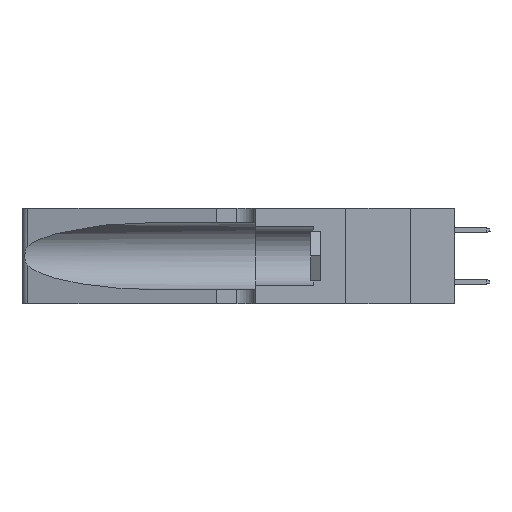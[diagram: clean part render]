
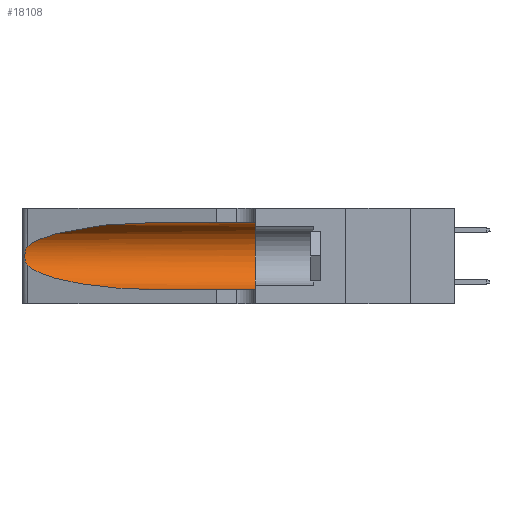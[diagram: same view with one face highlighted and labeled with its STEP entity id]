
A CAD part, left-side view. The second image highlights one B-rep face of the part: STEP entity #18108.
In plain terms, the highlighted cylindrical face has radius 3.308 mm (diameter 6.617 mm), a partial arc.
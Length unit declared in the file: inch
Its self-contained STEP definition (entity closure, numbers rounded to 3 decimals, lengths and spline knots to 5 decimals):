
#57 = CARTESIAN_POINT ( 'NONE',  ( 0.25487, 1.22718, 0.22369 ) ) ;
#286 = CARTESIAN_POINT ( 'NONE',  ( 0.26017, 1.23833, 0.17102 ) ) ;
#484 = CARTESIAN_POINT ( 'NONE',  ( 0.1305, 0.35, 0.31525 ) ) ;
#675 = ORIENTED_EDGE ( 'NONE', *, *, #28001, .F. ) ;
#751 = ORIENTED_EDGE ( 'NONE', *, *, #20551, .F. ) ;
#2755 = VERTEX_POINT ( 'NONE', #484 ) ;
#4154 = DIRECTION ( 'NONE',  ( 0., -1., 0. ) ) ;
#4269 = CARTESIAN_POINT ( 'NONE',  ( 0.25555, 1.22993, 0.14849 ) ) ;
#4335 = CARTESIAN_POINT ( 'NONE',  ( 0.1305, 0.72297, 0.05475 ) ) ;
#4946 = CARTESIAN_POINT ( 'NONE',  ( 0.25487, 1.22718, 0.14631 ) ) ;
#5287 = DIRECTION ( 'NONE',  ( 0., -1., 0. ) ) ;
#5870 = VERTEX_POINT ( 'NONE', #4335 ) ;
#6029 = CARTESIAN_POINT ( 'NONE',  ( 0.1305, 0.72297, 0.05475 ) ) ;
#6199 = CARTESIAN_POINT ( 'NONE',  ( 0.18966, 0.96281, 0.31525 ) ) ;
#7295 = CARTESIAN_POINT ( 'NONE',  ( 0.25854, 1.2359, 0.20912 ) ) ;
#7402 = ORIENTED_EDGE ( 'NONE', *, *, #29773, .T. ) ;
#7566 = DIRECTION ( 'NONE',  ( 0., -1., 0. ) ) ;
#8122 = VERTEX_POINT ( 'NONE', #38516 ) ;
#8570 = ORIENTED_EDGE ( 'NONE', *, *, #28626, .T. ) ;
#11115 = CYLINDRICAL_SURFACE ( 'NONE', #35770, 0.13025 ) ;
#11534 = EDGE_LOOP ( 'NONE', ( #14962, #7402, #8570, #28116, #751, #675 ) ) ;
#14216 = CARTESIAN_POINT ( 'NONE',  ( 0.25555, 1.22994, 0.2215 ) ) ;
#14439 = CARTESIAN_POINT ( 'NONE',  ( 0.25856, 1.23593, 0.16098 ) ) ;
#14962 = ORIENTED_EDGE ( 'NONE', *, *, #38275, .T. ) ;
#16842 = CARTESIAN_POINT ( 'NONE',  ( 0.2373, 1.15595, 0.28018 ) ) ;
#18108 = ADVANCED_FACE ( 'NONE', ( #24962 ), #11115, .F. ) ;
#18356 = CARTESIAN_POINT ( 'NONE',  ( 0.25639, 1.23186, 0.15144 ) ) ;
#20551 = EDGE_CURVE ( 'NONE', #2755, #45360, #32993, .T. ) ;
#21380 = CARTESIAN_POINT ( 'NONE',  ( 0.26018, 1.23835, 0.19895 ) ) ;
#22096 = LINE ( 'NONE', #28857, #41664 ) ;
#23373 = CARTESIAN_POINT ( 'NONE',  ( 0.25487, 1.22718, 0.14631 ) ) ;
#23606 = CARTESIAN_POINT ( 'NONE',  ( 0.18966, 0.96281, 0.05475 ) ) ;
#24962 = FACE_OUTER_BOUND ( 'NONE', #11534, .T. ) ;
#25114 = VECTOR ( 'NONE', #5287, 39.37008 ) ;
#25189 = CARTESIAN_POINT ( 'NONE',  ( 0.1305, 1.61858, 0.185 ) ) ;
#25211 = CARTESIAN_POINT ( 'NONE',  ( 0.1305, 0.35, 0.05475 ) ) ;
#25495 =( BOUNDED_CURVE ( )  B_SPLINE_CURVE ( 3, ( #23373, #41203, #23606, #6029 ),
 .UNSPECIFIED., .F., .F. ) 
 B_SPLINE_CURVE_WITH_KNOTS ( ( 4, 4 ),
 ( 3.44316, 4.71239 ),
 .UNSPECIFIED. ) 
 CURVE ( )  GEOMETRIC_REPRESENTATION_ITEM ( )  RATIONAL_B_SPLINE_CURVE ( ( 1., 0.87, 0.87, 1. ) ) 
 REPRESENTATION_ITEM ( '' )  );
#25879 = CARTESIAN_POINT ( 'NONE',  ( 0.1305, 1.61858, 0.05475 ) ) ;
#26024 =( BOUNDED_CURVE ( )  B_SPLINE_CURVE ( 3, ( #27270, #6199, #16842, #35340 ),
 .UNSPECIFIED., .F., .T. ) 
 B_SPLINE_CURVE_WITH_KNOTS ( ( 4, 4 ),
 ( 1.5708, 2.84003 ),
 .UNSPECIFIED. ) 
 CURVE ( )  GEOMETRIC_REPRESENTATION_ITEM ( )  RATIONAL_B_SPLINE_CURVE ( ( 1., 0.87, 0.87, 1. ) ) 
 REPRESENTATION_ITEM ( '' )  );
#27095 = AXIS2_PLACEMENT_3D ( 'NONE', #28658, #35576, #42754 ) ;
#27270 = CARTESIAN_POINT ( 'NONE',  ( 0.1305, 0.72297, 0.31525 ) ) ;
#27570 = VERTEX_POINT ( 'NONE', #33055 ) ;
#28001 = EDGE_CURVE ( 'NONE', #27570, #2755, #22096, .T. ) ;
#28116 = ORIENTED_EDGE ( 'NONE', *, *, #38051, .T. ) ;
#28626 = EDGE_CURVE ( 'NONE', #39001, #5870, #25495, .T. ) ;
#28658 = CARTESIAN_POINT ( 'NONE',  ( 0.1305, 0.35, 0.185 ) ) ;
#28857 = CARTESIAN_POINT ( 'NONE',  ( 0.1305, 1.61858, 0.31525 ) ) ;
#29773 = EDGE_CURVE ( 'NONE', #8122, #39001, #36017, .T. ) ;
#32044 = CARTESIAN_POINT ( 'NONE',  ( 0.26075, 1.23896, 0.178 ) ) ;
#32993 = CIRCLE ( 'NONE', #27095, 0.13025 ) ;
#33055 = CARTESIAN_POINT ( 'NONE',  ( 0.1305, 0.72297, 0.31525 ) ) ;
#35340 = CARTESIAN_POINT ( 'NONE',  ( 0.25487, 1.22718, 0.22369 ) ) ;
#35503 = CARTESIAN_POINT ( 'NONE',  ( 0.26075, 1.23896, 0.19203 ) ) ;
#35576 = DIRECTION ( 'NONE',  ( 0., 1., 0. ) ) ;
#35770 = AXIS2_PLACEMENT_3D ( 'NONE', #25189, #4154, #39536 ) ;
#36017 = B_SPLINE_CURVE_WITH_KNOTS ( 'NONE', 3,
 ( #57, #14216, #42454, #38981, #7295, #21380, #35503, #32044, #286, #14439, #39204, #18356, #4269, #4946 ),
 .UNSPECIFIED., .F., .F.,
 ( 4, 2, 2, 2, 2, 2, 4 ),
 ( 0., 0.00027, 0.00053, 0.00107, 0.0016, 0.00187, 0.00214 ),
 .UNSPECIFIED. ) ;
#38051 = EDGE_CURVE ( 'NONE', #5870, #45360, #40923, .T. ) ;
#38275 = EDGE_CURVE ( 'NONE', #27570, #8122, #26024, .T. ) ;
#38516 = CARTESIAN_POINT ( 'NONE',  ( 0.25487, 1.22718, 0.22369 ) ) ;
#38981 = CARTESIAN_POINT ( 'NONE',  ( 0.25787, 1.23484, 0.2124 ) ) ;
#39001 = VERTEX_POINT ( 'NONE', #44677 ) ;
#39204 = CARTESIAN_POINT ( 'NONE',  ( 0.25789, 1.23486, 0.15765 ) ) ;
#39536 = DIRECTION ( 'NONE',  ( 0., 0., -1. ) ) ;
#40923 = LINE ( 'NONE', #25879, #25114 ) ;
#41203 = CARTESIAN_POINT ( 'NONE',  ( 0.2373, 1.15595, 0.08982 ) ) ;
#41664 = VECTOR ( 'NONE', #7566, 39.37008 ) ;
#42454 = CARTESIAN_POINT ( 'NONE',  ( 0.25639, 1.23184, 0.21858 ) ) ;
#42754 = DIRECTION ( 'NONE',  ( 0., 0., 1. ) ) ;
#44677 = CARTESIAN_POINT ( 'NONE',  ( 0.25487, 1.22718, 0.14631 ) ) ;
#45360 = VERTEX_POINT ( 'NONE', #25211 ) ;
